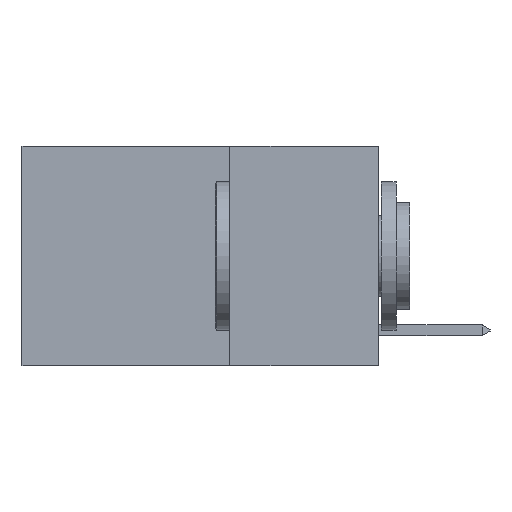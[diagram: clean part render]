
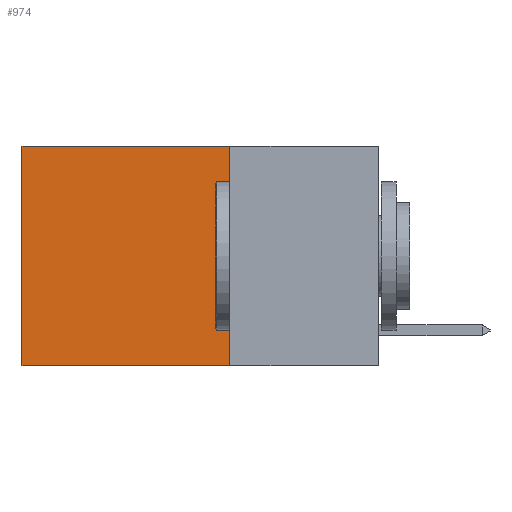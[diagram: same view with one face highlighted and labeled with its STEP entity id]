
A CAD part, left-side view. The second image highlights one B-rep face of the part: STEP entity #974.
In plain terms, the highlighted planar face has unit normal (-1, 0, 0).
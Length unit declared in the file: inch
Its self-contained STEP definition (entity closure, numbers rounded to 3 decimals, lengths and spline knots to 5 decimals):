
#645 = ORIENTED_EDGE ( 'NONE', *, *, #4303, .F. ) ;
#743 = CARTESIAN_POINT ( 'NONE',  ( 0.2625, 0.25, -0.37 ) ) ;
#974 = ADVANCED_FACE ( 'NONE', ( #5624 ), #4733, .F. ) ;
#1356 = CARTESIAN_POINT ( 'NONE',  ( 0.2625, 0.25, -0.37 ) ) ;
#1443 = LINE ( 'NONE', #743, #3670 ) ;
#1545 = EDGE_CURVE ( 'NONE', #9277, #10770, #6368, .T. ) ;
#1691 = ORIENTED_EDGE ( 'NONE', *, *, #8359, .F. ) ;
#2635 = DIRECTION ( 'NONE',  ( 0., 1., 0. ) ) ;
#2871 = CARTESIAN_POINT ( 'NONE',  ( 0.2625, 0.6, -0.37 ) ) ;
#3126 = CARTESIAN_POINT ( 'NONE',  ( 0.2625, 0.25, 0. ) ) ;
#3334 = LINE ( 'NONE', #11598, #5839 ) ;
#3670 = VECTOR ( 'NONE', #2635, 39.37008 ) ;
#3839 = VECTOR ( 'NONE', #7311, 39.37008 ) ;
#3861 = AXIS2_PLACEMENT_3D ( 'NONE', #9449, #9365, #9205 ) ;
#4156 = CARTESIAN_POINT ( 'NONE',  ( 0.2625, 0.6, 0. ) ) ;
#4303 = EDGE_CURVE ( 'NONE', #9277, #5560, #3334, .T. ) ;
#4733 = PLANE ( 'NONE',  #3861 ) ;
#5257 = EDGE_LOOP ( 'NONE', ( #10149, #1691, #645, #8303 ) ) ;
#5560 = VERTEX_POINT ( 'NONE', #1356 ) ;
#5624 = FACE_OUTER_BOUND ( 'NONE', #5257, .T. ) ;
#5839 = VECTOR ( 'NONE', #11597, 39.37008 ) ;
#6368 = LINE ( 'NONE', #7465, #3839 ) ;
#6941 = EDGE_CURVE ( 'NONE', #10770, #11935, #9139, .T. ) ;
#7311 = DIRECTION ( 'NONE',  ( 0., 1., 0. ) ) ;
#7465 = CARTESIAN_POINT ( 'NONE',  ( 0.2625, 0.25, 0. ) ) ;
#8303 = ORIENTED_EDGE ( 'NONE', *, *, #1545, .T. ) ;
#8359 = EDGE_CURVE ( 'NONE', #5560, #11935, #1443, .T. ) ;
#9139 = LINE ( 'NONE', #4156, #11316 ) ;
#9205 = DIRECTION ( 'NONE',  ( 0., 0., -1. ) ) ;
#9277 = VERTEX_POINT ( 'NONE', #3126 ) ;
#9365 = DIRECTION ( 'NONE',  ( 1., 0., 0. ) ) ;
#9449 = CARTESIAN_POINT ( 'NONE',  ( 0.2625, 0.25, 0. ) ) ;
#9761 = DIRECTION ( 'NONE',  ( 0., 0., -1. ) ) ;
#10149 = ORIENTED_EDGE ( 'NONE', *, *, #6941, .T. ) ;
#10770 = VERTEX_POINT ( 'NONE', #10992 ) ;
#10992 = CARTESIAN_POINT ( 'NONE',  ( 0.2625, 0.6, 0. ) ) ;
#11316 = VECTOR ( 'NONE', #9761, 39.37008 ) ;
#11597 = DIRECTION ( 'NONE',  ( 0., 0., -1. ) ) ;
#11598 = CARTESIAN_POINT ( 'NONE',  ( 0.2625, 0.25, 0. ) ) ;
#11935 = VERTEX_POINT ( 'NONE', #2871 ) ;
